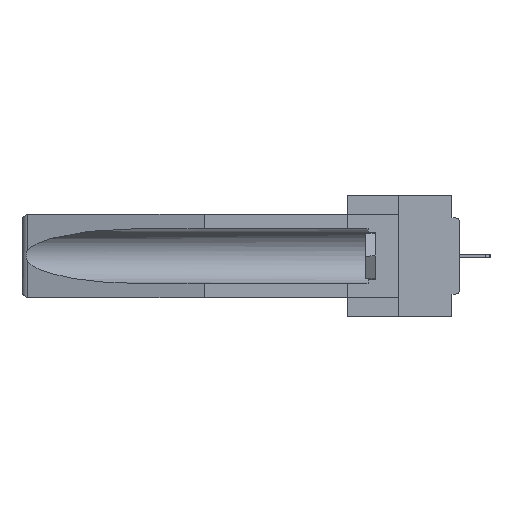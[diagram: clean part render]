
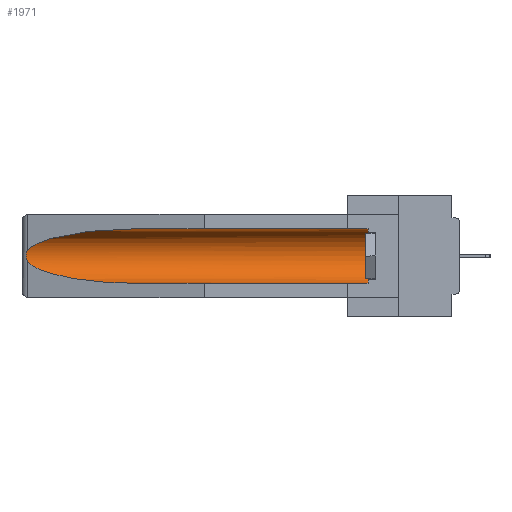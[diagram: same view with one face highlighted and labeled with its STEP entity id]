
A CAD part, left-side view. The second image highlights one B-rep face of the part: STEP entity #1971.
In plain terms, the highlighted cylindrical face has radius 2.857 mm (diameter 5.715 mm), a partial arc.
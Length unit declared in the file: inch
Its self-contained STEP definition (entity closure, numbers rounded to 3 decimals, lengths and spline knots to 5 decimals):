
#485 = DIRECTION ( 'NONE',  ( 0., 0., 1. ) ) ;
#771 = AXIS2_PLACEMENT_3D ( 'NONE', #14310, #25414, #485 ) ;
#1139 = CARTESIAN_POINT ( 'NONE',  ( 0.155, 0.126, -0.059 ) ) ;
#1148 = CYLINDRICAL_SURFACE ( 'NONE', #27285, 0.1125 ) ;
#1926 = CARTESIAN_POINT ( 'NONE',  ( 0.2675, 1.53308, -0.17534 ) ) ;
#1971 = ADVANCED_FACE ( 'NONE', ( #25919 ), #1148, .F. ) ;
#2422 = ORIENTED_EDGE ( 'NONE', *, *, #21066, .T. ) ;
#2579 =( BOUNDED_CURVE ( )  B_SPLINE_CURVE ( 3, ( #6532, #14914, #31429, #17617 ),
 .UNSPECIFIED., .F., .T. ) 
 B_SPLINE_CURVE_WITH_KNOTS ( ( 4, 4 ),
 ( 4.71239, 6.08839 ),
 .UNSPECIFIED. ) 
 CURVE ( )  GEOMETRIC_REPRESENTATION_ITEM ( )  RATIONAL_B_SPLINE_CURVE ( ( 1., 0.848, 0.848, 1. ) ) 
 REPRESENTATION_ITEM ( '' )  );
#3755 = VECTOR ( 'NONE', #26964, 39.37008 ) ;
#3987 = CARTESIAN_POINT ( 'NONE',  ( 0.155, 1.07973, -0.059 ) ) ;
#5059 = CARTESIAN_POINT ( 'NONE',  ( 0.155, 1.07973, -0.284 ) ) ;
#5298 = VERTEX_POINT ( 'NONE', #16577 ) ;
#6098 = ORIENTED_EDGE ( 'NONE', *, *, #28386, .T. ) ;
#6532 = CARTESIAN_POINT ( 'NONE',  ( 0.155, 1.07973, -0.059 ) ) ;
#7256 = ORIENTED_EDGE ( 'NONE', *, *, #23874, .T. ) ;
#7363 = DIRECTION ( 'NONE',  ( 0., 1., 0. ) ) ;
#7415 = CARTESIAN_POINT ( 'NONE',  ( 0.26655, 1.53094, -0.18657 ) ) ;
#8249 = EDGE_CURVE ( 'NONE', #24552, #19063, #12940, .T. ) ;
#10711 = ORIENTED_EDGE ( 'NONE', *, *, #8249, .T. ) ;
#12940 = LINE ( 'NONE', #35139, #3755 ) ;
#13227 = CARTESIAN_POINT ( 'NONE',  ( 0.26597, 1.52961, -0.15275 ) ) ;
#13502 = VERTEX_POINT ( 'NONE', #29137 ) ;
#14310 = CARTESIAN_POINT ( 'NONE',  ( 0.155, 0.126, -0.1715 ) ) ;
#14914 = CARTESIAN_POINT ( 'NONE',  ( 0.21114, 1.30732, -0.059 ) ) ;
#15097 = EDGE_LOOP ( 'NONE', ( #2422, #7256, #30280, #25461, #6098, #10711 ) ) ;
#15553 = LINE ( 'NONE', #34976, #28038 ) ;
#15760 = CARTESIAN_POINT ( 'NONE',  ( 0.2675, 1.53308, -0.16763 ) ) ;
#16020 = VERTEX_POINT ( 'NONE', #32486 ) ;
#16051 = EDGE_CURVE ( 'NONE', #16020, #18287, #16497, .T. ) ;
#16497 =( BOUNDED_CURVE ( )  B_SPLINE_CURVE ( 3, ( #26517, #29941, #24303, #5059 ),
 .UNSPECIFIED., .F., .F. ) 
 B_SPLINE_CURVE_WITH_KNOTS ( ( 4, 4 ),
 ( 0.1948, 1.5708 ),
 .UNSPECIFIED. ) 
 CURVE ( )  GEOMETRIC_REPRESENTATION_ITEM ( )  RATIONAL_B_SPLINE_CURVE ( ( 1., 0.848, 0.848, 1. ) ) 
 REPRESENTATION_ITEM ( '' )  );
#16577 = CARTESIAN_POINT ( 'NONE',  ( 0.26537, 1.52718, -0.14972 ) ) ;
#17617 = CARTESIAN_POINT ( 'NONE',  ( 0.26537, 1.52718, -0.14972 ) ) ;
#18287 = VERTEX_POINT ( 'NONE', #19286 ) ;
#18480 = CARTESIAN_POINT ( 'NONE',  ( 0.26597, 1.5296, -0.19026 ) ) ;
#19063 = VERTEX_POINT ( 'NONE', #3987 ) ;
#19286 = CARTESIAN_POINT ( 'NONE',  ( 0.155, 1.07973, -0.284 ) ) ;
#21066 = EDGE_CURVE ( 'NONE', #19063, #5298, #2579, .T. ) ;
#21664 = CIRCLE ( 'NONE', #771, 0.1125 ) ;
#23874 = EDGE_CURVE ( 'NONE', #5298, #16020, #31624, .T. ) ;
#24303 = CARTESIAN_POINT ( 'NONE',  ( 0.21114, 1.30732, -0.284 ) ) ;
#24312 = CARTESIAN_POINT ( 'NONE',  ( 0.2673, 1.53269, -0.17917 ) ) ;
#24490 = CARTESIAN_POINT ( 'NONE',  ( 0.26537, 1.52718, -0.19328 ) ) ;
#24552 = VERTEX_POINT ( 'NONE', #1139 ) ;
#25414 = DIRECTION ( 'NONE',  ( 0., -1., 0. ) ) ;
#25461 = ORIENTED_EDGE ( 'NONE', *, *, #32367, .F. ) ;
#25919 = FACE_OUTER_BOUND ( 'NONE', #15097, .T. ) ;
#26517 = CARTESIAN_POINT ( 'NONE',  ( 0.26537, 1.52718, -0.19328 ) ) ;
#26964 = DIRECTION ( 'NONE',  ( 0., 1., 0. ) ) ;
#27231 = CARTESIAN_POINT ( 'NONE',  ( 0.26654, 1.53092, -0.15636 ) ) ;
#27285 = AXIS2_PLACEMENT_3D ( 'NONE', #30986, #34255, #31179 ) ;
#28038 = VECTOR ( 'NONE', #7363, 39.37008 ) ;
#28386 = EDGE_CURVE ( 'NONE', #13502, #24552, #21664, .T. ) ;
#29137 = CARTESIAN_POINT ( 'NONE',  ( 0.155, 0.126, -0.284 ) ) ;
#29941 = CARTESIAN_POINT ( 'NONE',  ( 0.25451, 1.48313, -0.24835 ) ) ;
#30280 = ORIENTED_EDGE ( 'NONE', *, *, #16051, .T. ) ;
#30986 = CARTESIAN_POINT ( 'NONE',  ( 0.155, -0.30754, -0.1715 ) ) ;
#31179 = DIRECTION ( 'NONE',  ( 0., 0., 1. ) ) ;
#31429 = CARTESIAN_POINT ( 'NONE',  ( 0.25451, 1.48313, -0.09465 ) ) ;
#31624 = B_SPLINE_CURVE_WITH_KNOTS ( 'NONE', 3,
 ( #32329, #13227, #27231, #35231, #15760, #1926, #24312, #7415, #18480, #24490 ),
 .UNSPECIFIED., .F., .F.,
 ( 4, 2, 2, 2, 4 ),
 ( 0., 0.00029, 0.00058, 0.00087, 0.00117 ),
 .UNSPECIFIED. ) ;
#32329 = CARTESIAN_POINT ( 'NONE',  ( 0.26537, 1.52718, -0.14972 ) ) ;
#32367 = EDGE_CURVE ( 'NONE', #13502, #18287, #15553, .T. ) ;
#32486 = CARTESIAN_POINT ( 'NONE',  ( 0.26537, 1.52718, -0.19328 ) ) ;
#34255 = DIRECTION ( 'NONE',  ( 0., 1., 0. ) ) ;
#34976 = CARTESIAN_POINT ( 'NONE',  ( 0.155, -0.30754, -0.284 ) ) ;
#35139 = CARTESIAN_POINT ( 'NONE',  ( 0.155, -0.30754, -0.059 ) ) ;
#35231 = CARTESIAN_POINT ( 'NONE',  ( 0.2673, 1.5327, -0.16383 ) ) ;
